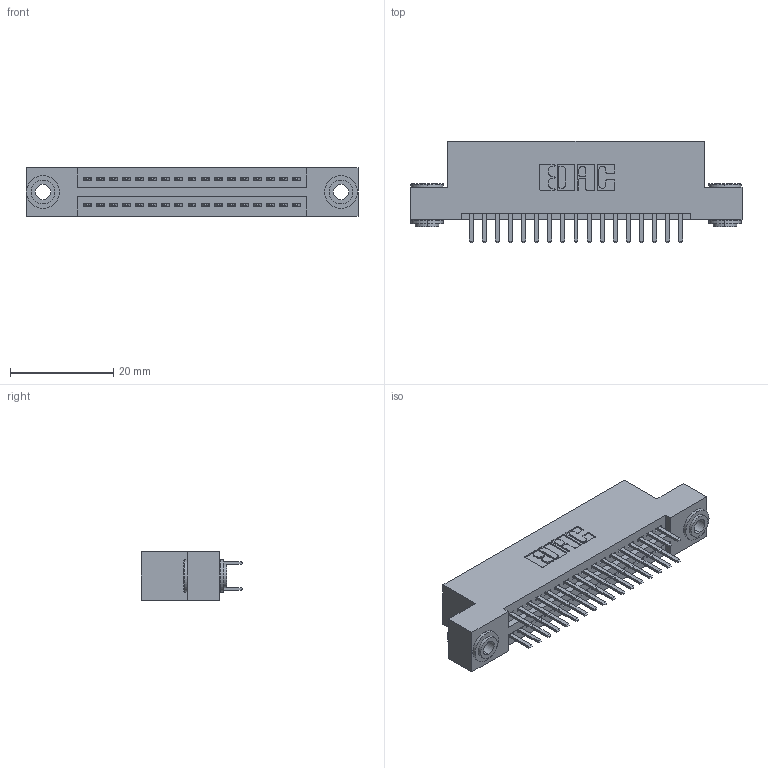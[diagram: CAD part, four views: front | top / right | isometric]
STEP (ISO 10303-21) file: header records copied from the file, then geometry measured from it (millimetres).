
FILE_DESCRIPTION (( 'STEP AP203' ), '1' );
FILE_NAME ('345-034-520-203.STEP', '2019-10-28T05:49:35', ( '' ), ( '' ), 'SwSTEP 2.0', 'SolidWorks 2016', '' );
FILE_SCHEMA (( 'CONFIG_CONTROL_DESIGN' ));
Length unit declared in the file: inch
Products named in the file (4): 345-250-002_345-250-002-102; 345-034-520-203; 345-292-001_345-293-120; 345 Part_Flush Mounting Lugs - 0.156 Dia-TH
Assembly tree (37 placements, depth 2):
  345-034-520-203
    345 Part_Flush Mounting Lugs - 0.156 Dia-TH
    345-292-001_345-293-120  x34
    345-250-002_345-250-002-102  x2
Bounding box: 64.39 x 19.68 x 9.4 mm (x, y, z)
Volume: 6027.2 mm3; surface area: 8598.1 mm2
Topology: 37 solids, 37 shells, 2000 faces, 5755 edges, 3742 vertices
Faces by surface type: plane 1280, cylinder 712, cone 8
Entity records: 17468 total; most frequent: CARTESIAN_POINT 2939, ORIENTED_EDGE 2854, DIRECTION 2641, EDGE_CURVE 1427, VECTOR 1199, LINE 1199, VERTEX_POINT 946, AXIS2_PLACEMENT_3D 721
